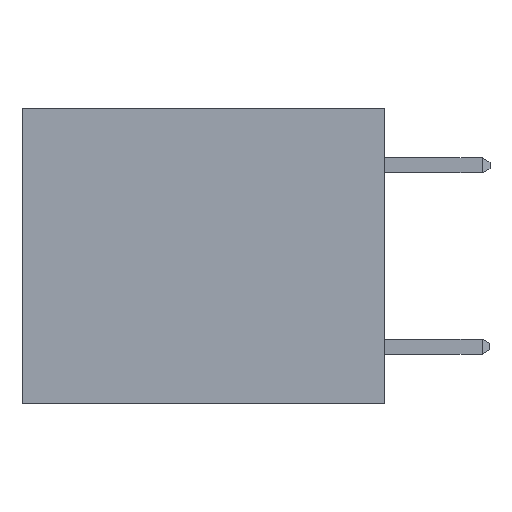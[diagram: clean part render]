
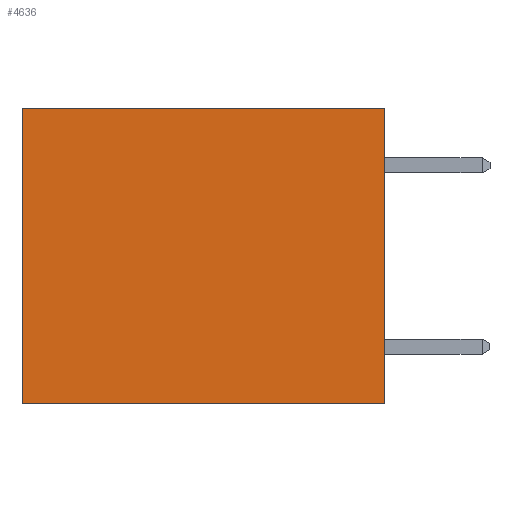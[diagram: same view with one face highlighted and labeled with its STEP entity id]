
A CAD part, left-side view. The second image highlights one B-rep face of the part: STEP entity #4636.
In plain terms, the highlighted planar face has unit normal (-1, 0, 0).
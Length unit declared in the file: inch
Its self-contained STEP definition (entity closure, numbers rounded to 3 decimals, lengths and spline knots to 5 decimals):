
#201 = VECTOR ( 'NONE', #8106, 39.37008 ) ;
#417 = PLANE ( 'NONE',  #4033 ) ;
#1689 = CARTESIAN_POINT ( 'NONE',  ( 0.3165, 0., 0. ) ) ;
#1923 = EDGE_CURVE ( 'NONE', #2308, #8571, #5510, .T. ) ;
#2191 = LINE ( 'NONE', #6178, #201 ) ;
#2308 = VERTEX_POINT ( 'NONE', #3436 ) ;
#2317 = DIRECTION ( 'NONE',  ( 0., 0., -1. ) ) ;
#2433 = ORIENTED_EDGE ( 'NONE', *, *, #8409, .F. ) ;
#2511 = LINE ( 'NONE', #6221, #8472 ) ;
#3000 = DIRECTION ( 'NONE',  ( 1., 0., 0. ) ) ;
#3436 = CARTESIAN_POINT ( 'NONE',  ( 0.3165, 0.6, 0. ) ) ;
#3774 = EDGE_LOOP ( 'NONE', ( #4286, #7205, #2433, #5156 ) ) ;
#4033 = AXIS2_PLACEMENT_3D ( 'NONE', #7076, #3000, #7765 ) ;
#4086 = VERTEX_POINT ( 'NONE', #4296 ) ;
#4097 = DIRECTION ( 'NONE',  ( 0., 1., 0. ) ) ;
#4166 = CARTESIAN_POINT ( 'NONE',  ( 0.3165, 0.6, -0.49 ) ) ;
#4189 = EDGE_CURVE ( 'NONE', #4086, #2308, #6032, .T. ) ;
#4286 = ORIENTED_EDGE ( 'NONE', *, *, #1923, .T. ) ;
#4296 = CARTESIAN_POINT ( 'NONE',  ( 0.3165, 0., 0. ) ) ;
#4636 = ADVANCED_FACE ( 'NONE', ( #8465 ), #417, .F. ) ;
#5156 = ORIENTED_EDGE ( 'NONE', *, *, #4189, .T. ) ;
#5510 = LINE ( 'NONE', #6402, #6278 ) ;
#6032 = LINE ( 'NONE', #1689, #6237 ) ;
#6178 = CARTESIAN_POINT ( 'NONE',  ( 0.3165, 0., -0.49 ) ) ;
#6221 = CARTESIAN_POINT ( 'NONE',  ( 0.3165, 0., -0.49 ) ) ;
#6237 = VECTOR ( 'NONE', #7152, 39.37008 ) ;
#6278 = VECTOR ( 'NONE', #2317, 39.37008 ) ;
#6402 = CARTESIAN_POINT ( 'NONE',  ( 0.3165, 0.6, -0.49 ) ) ;
#6618 = EDGE_CURVE ( 'NONE', #8212, #8571, #2511, .T. ) ;
#7076 = CARTESIAN_POINT ( 'NONE',  ( 0.3165, 0., -0.49 ) ) ;
#7152 = DIRECTION ( 'NONE',  ( 0., 1., 0. ) ) ;
#7205 = ORIENTED_EDGE ( 'NONE', *, *, #6618, .F. ) ;
#7765 = DIRECTION ( 'NONE',  ( 0., 0., -1. ) ) ;
#8106 = DIRECTION ( 'NONE',  ( 0., 0., -1. ) ) ;
#8212 = VERTEX_POINT ( 'NONE', #8248 ) ;
#8248 = CARTESIAN_POINT ( 'NONE',  ( 0.3165, 0., -0.49 ) ) ;
#8409 = EDGE_CURVE ( 'NONE', #4086, #8212, #2191, .T. ) ;
#8465 = FACE_OUTER_BOUND ( 'NONE', #3774, .T. ) ;
#8472 = VECTOR ( 'NONE', #4097, 39.37008 ) ;
#8571 = VERTEX_POINT ( 'NONE', #4166 ) ;
